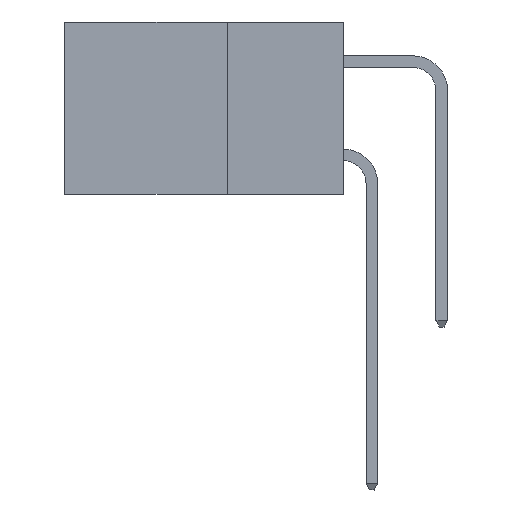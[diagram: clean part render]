
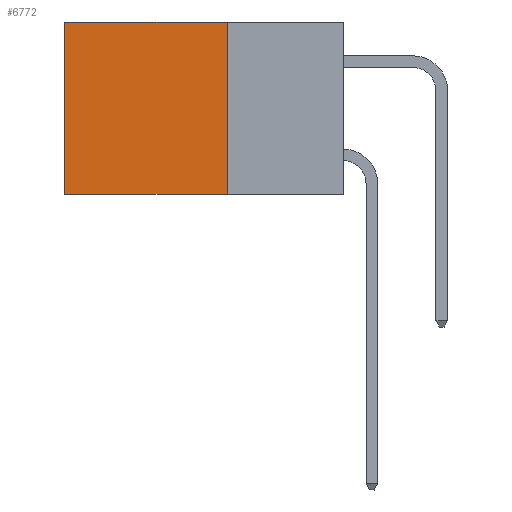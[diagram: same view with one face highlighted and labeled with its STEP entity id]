
A CAD part, left-side view. The second image highlights one B-rep face of the part: STEP entity #6772.
In plain terms, the highlighted planar face has unit normal (-1, 0, 0).
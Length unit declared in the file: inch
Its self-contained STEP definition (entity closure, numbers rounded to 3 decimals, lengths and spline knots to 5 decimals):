
#209 = FACE_OUTER_BOUND ( 'NONE', #5572, .T. ) ;
#530 = CARTESIAN_POINT ( 'NONE',  ( 0.2615, 0.25, -0.37 ) ) ;
#648 = CARTESIAN_POINT ( 'NONE',  ( 0.2615, 0.25, -0.37 ) ) ;
#1365 = DIRECTION ( 'NONE',  ( 1., 0., 0. ) ) ;
#1674 = DIRECTION ( 'NONE',  ( 0., 1., 0. ) ) ;
#1778 = VECTOR ( 'NONE', #1674, 39.37008 ) ;
#2958 = ORIENTED_EDGE ( 'NONE', *, *, #9471, .T. ) ;
#3253 = CARTESIAN_POINT ( 'NONE',  ( 0.2615, 0.25, -0.37 ) ) ;
#3402 = EDGE_CURVE ( 'NONE', #11924, #10523, #5946, .T. ) ;
#3631 = VECTOR ( 'NONE', #4903, 39.37008 ) ;
#3929 = CARTESIAN_POINT ( 'NONE',  ( 0.2615, 0.25, 0. ) ) ;
#4763 = EDGE_CURVE ( 'NONE', #11924, #5693, #7329, .T. ) ;
#4903 = DIRECTION ( 'NONE',  ( 0., 0., -1. ) ) ;
#5439 = CARTESIAN_POINT ( 'NONE',  ( 0.2615, 0.25, 0. ) ) ;
#5501 = LINE ( 'NONE', #9857, #13815 ) ;
#5572 = EDGE_LOOP ( 'NONE', ( #2958, #10671, #13050, #11745 ) ) ;
#5693 = VERTEX_POINT ( 'NONE', #5910 ) ;
#5910 = CARTESIAN_POINT ( 'NONE',  ( 0.2615, 0.6, 0. ) ) ;
#5946 = LINE ( 'NONE', #530, #3631 ) ;
#6772 = ADVANCED_FACE ( 'NONE', ( #209 ), #11295, .F. ) ;
#7329 = LINE ( 'NONE', #3929, #1778 ) ;
#7705 = DIRECTION ( 'NONE',  ( 0., 1., 0. ) ) ;
#8682 = LINE ( 'NONE', #3253, #13188 ) ;
#9378 = VERTEX_POINT ( 'NONE', #14037 ) ;
#9471 = EDGE_CURVE ( 'NONE', #5693, #9378, #5501, .T. ) ;
#9857 = CARTESIAN_POINT ( 'NONE',  ( 0.2615, 0.6, -0.37 ) ) ;
#10008 = CARTESIAN_POINT ( 'NONE',  ( 0.2615, 0.25, -0.37 ) ) ;
#10523 = VERTEX_POINT ( 'NONE', #648 ) ;
#10671 = ORIENTED_EDGE ( 'NONE', *, *, #10718, .F. ) ;
#10718 = EDGE_CURVE ( 'NONE', #10523, #9378, #8682, .T. ) ;
#11056 = DIRECTION ( 'NONE',  ( 0., 0., -1. ) ) ;
#11295 = PLANE ( 'NONE',  #11867 ) ;
#11745 = ORIENTED_EDGE ( 'NONE', *, *, #4763, .T. ) ;
#11867 = AXIS2_PLACEMENT_3D ( 'NONE', #10008, #1365, #13472 ) ;
#11924 = VERTEX_POINT ( 'NONE', #5439 ) ;
#13050 = ORIENTED_EDGE ( 'NONE', *, *, #3402, .F. ) ;
#13188 = VECTOR ( 'NONE', #7705, 39.37008 ) ;
#13472 = DIRECTION ( 'NONE',  ( 0., 0., -1. ) ) ;
#13815 = VECTOR ( 'NONE', #11056, 39.37008 ) ;
#14037 = CARTESIAN_POINT ( 'NONE',  ( 0.2615, 0.6, -0.37 ) ) ;
